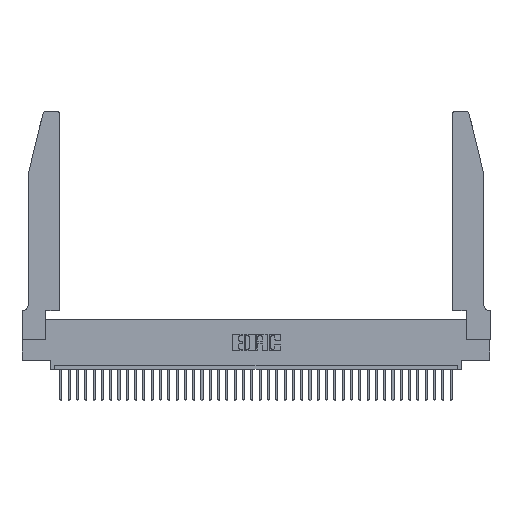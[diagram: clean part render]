
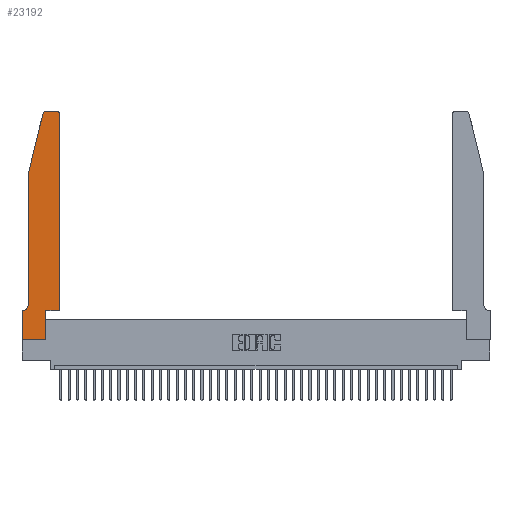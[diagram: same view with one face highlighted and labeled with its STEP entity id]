
A CAD part, top view. The second image highlights one B-rep face of the part: STEP entity #23192.
In plain terms, the highlighted planar face has unit normal (0, 0, 1).
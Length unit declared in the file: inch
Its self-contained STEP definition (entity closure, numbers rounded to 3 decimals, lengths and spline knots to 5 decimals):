
#135 = EDGE_CURVE ( 'NONE', #16836, #17390, #16397, .T. ) ;
#610 = DIRECTION ( 'NONE',  ( 1., 0., 0. ) ) ;
#1029 = DIRECTION ( 'NONE',  ( 0., -1., 0. ) ) ;
#2072 = ORIENTED_EDGE ( 'NONE', *, *, #16453, .T. ) ;
#3809 = EDGE_CURVE ( 'NONE', #31305, #38324, #21868, .T. ) ;
#4408 = AXIS2_PLACEMENT_3D ( 'NONE', #30358, #13214, #38181 ) ;
#4433 = ORIENTED_EDGE ( 'NONE', *, *, #30087, .T. ) ;
#4490 = EDGE_CURVE ( 'NONE', #38324, #21336, #21433, .T. ) ;
#5749 = ORIENTED_EDGE ( 'NONE', *, *, #23610, .T. ) ;
#5936 = LINE ( 'NONE', #21423, #18522 ) ;
#6411 = VECTOR ( 'NONE', #39731, 39.37008 ) ;
#6903 = VERTEX_POINT ( 'NONE', #28206 ) ;
#7872 = CARTESIAN_POINT ( 'NONE',  ( 0.25487, 2.72718, 0.37 ) ) ;
#8053 = CARTESIAN_POINT ( 'NONE',  ( 0., 0., 0.37 ) ) ;
#8839 = LINE ( 'NONE', #24676, #6411 ) ;
#9004 = VECTOR ( 'NONE', #610, 39.37008 ) ;
#9751 = CARTESIAN_POINT ( 'NONE',  ( 0.2605, 2.75, 0.37 ) ) ;
#9951 = AXIS2_PLACEMENT_3D ( 'NONE', #19405, #22533, #25153 ) ;
#10279 = VECTOR ( 'NONE', #39631, 39.37008 ) ;
#10837 = LINE ( 'NONE', #33483, #38509 ) ;
#10920 = FACE_OUTER_BOUND ( 'NONE', #16718, .T. ) ;
#11828 = EDGE_CURVE ( 'NONE', #39934, #39198, #5936, .T. ) ;
#13186 = VERTEX_POINT ( 'NONE', #14223 ) ;
#13214 = DIRECTION ( 'NONE',  ( 0., 0., -1. ) ) ;
#13774 = ORIENTED_EDGE ( 'NONE', *, *, #4490, .T. ) ;
#14223 = CARTESIAN_POINT ( 'NONE',  ( 0., 0.35, 0.37 ) ) ;
#15357 = CARTESIAN_POINT ( 'NONE',  ( 0.0755, 0.42, 0.37 ) ) ;
#16397 = CIRCLE ( 'NONE', #4408, 0.07 ) ;
#16434 = AXIS2_PLACEMENT_3D ( 'NONE', #36152, #20536, #32937 ) ;
#16453 = EDGE_CURVE ( 'NONE', #6903, #18025, #40066, .T. ) ;
#16718 = EDGE_LOOP ( 'NONE', ( #21951, #13774, #36897, #24852, #38712, #35125, #4433, #31146, #17960, #5749, #2072, #26581 ) ) ;
#16836 = VERTEX_POINT ( 'NONE', #15357 ) ;
#16858 = DIRECTION ( 'NONE',  ( 1., 0., 0. ) ) ;
#17140 = DIRECTION ( 'NONE',  ( 0., 0., 1. ) ) ;
#17390 = VERTEX_POINT ( 'NONE', #38244 ) ;
#17960 = ORIENTED_EDGE ( 'NONE', *, *, #11828, .T. ) ;
#18025 = VERTEX_POINT ( 'NONE', #33419 ) ;
#18165 = DIRECTION ( 'NONE',  ( 1., 0., 0. ) ) ;
#18201 = LINE ( 'NONE', #31940, #9004 ) ;
#18522 = VECTOR ( 'NONE', #24600, 39.37008 ) ;
#19405 = CARTESIAN_POINT ( 'NONE',  ( 0., 0.35, 0.37 ) ) ;
#19458 = VECTOR ( 'NONE', #34037, 39.37008 ) ;
#20536 = DIRECTION ( 'NONE',  ( 0., 0., 1. ) ) ;
#20901 = LINE ( 'NONE', #21155, #10279 ) ;
#21155 = CARTESIAN_POINT ( 'NONE',  ( 0.0755, 2., 0.37 ) ) ;
#21336 = VERTEX_POINT ( 'NONE', #7872 ) ;
#21423 = CARTESIAN_POINT ( 'NONE',  ( 0.2865, 0.35, 0.37 ) ) ;
#21433 = CIRCLE ( 'NONE', #16434, 0.03 ) ;
#21868 = LINE ( 'NONE', #9751, #19458 ) ;
#21951 = ORIENTED_EDGE ( 'NONE', *, *, #3809, .T. ) ;
#22125 = PLANE ( 'NONE',  #9951 ) ;
#22296 = CARTESIAN_POINT ( 'NONE',  ( 0., 0., 0.37 ) ) ;
#22533 = DIRECTION ( 'NONE',  ( 0., 0., 1. ) ) ;
#22954 = EDGE_CURVE ( 'NONE', #25829, #39934, #18201, .T. ) ;
#23192 = ADVANCED_FACE ( 'NONE', ( #10920 ), #22125, .T. ) ;
#23610 = EDGE_CURVE ( 'NONE', #39198, #6903, #10837, .T. ) ;
#23915 = DIRECTION ( 'NONE',  ( 0., 1., 0. ) ) ;
#24600 = DIRECTION ( 'NONE',  ( 0., 1., 0. ) ) ;
#24676 = CARTESIAN_POINT ( 'NONE',  ( 0.0755, 0.35, 0.37 ) ) ;
#24852 = ORIENTED_EDGE ( 'NONE', *, *, #33521, .T. ) ;
#25153 = DIRECTION ( 'NONE',  ( 1., 0., 0. ) ) ;
#25257 = EDGE_CURVE ( 'NONE', #21336, #33559, #32673, .T. ) ;
#25829 = VERTEX_POINT ( 'NONE', #8053 ) ;
#26127 = CARTESIAN_POINT ( 'NONE',  ( 0.284, 2.75, 0.37 ) ) ;
#26581 = ORIENTED_EDGE ( 'NONE', *, *, #28213, .T. ) ;
#27430 = VECTOR ( 'NONE', #23915, 39.37008 ) ;
#28206 = CARTESIAN_POINT ( 'NONE',  ( 0.4505, 0.35, 0.37 ) ) ;
#28213 = EDGE_CURVE ( 'NONE', #18025, #31305, #38814, .T. ) ;
#28311 = VECTOR ( 'NONE', #39854, 39.37008 ) ;
#30087 = EDGE_CURVE ( 'NONE', #13186, #25829, #34750, .T. ) ;
#30358 = CARTESIAN_POINT ( 'NONE',  ( 0.0055, 0.42, 0.37 ) ) ;
#30397 = CARTESIAN_POINT ( 'NONE',  ( 0.2865, 0.35, 0.37 ) ) ;
#31146 = ORIENTED_EDGE ( 'NONE', *, *, #22954, .T. ) ;
#31305 = VERTEX_POINT ( 'NONE', #38237 ) ;
#31940 = CARTESIAN_POINT ( 'NONE',  ( 0., 0., 0.37 ) ) ;
#32021 = CARTESIAN_POINT ( 'NONE',  ( 0.4205, 2.72, 0.37 ) ) ;
#32536 = CARTESIAN_POINT ( 'NONE',  ( 0.4505, 0.35, 0.37 ) ) ;
#32673 = LINE ( 'NONE', #39723, #28311 ) ;
#32674 = CARTESIAN_POINT ( 'NONE',  ( 0.0755, 2., 0.37 ) ) ;
#32719 = EDGE_CURVE ( 'NONE', #17390, #13186, #8839, .T. ) ;
#32937 = DIRECTION ( 'NONE',  ( 1., 0., 0. ) ) ;
#33419 = CARTESIAN_POINT ( 'NONE',  ( 0.4505, 2.72, 0.37 ) ) ;
#33483 = CARTESIAN_POINT ( 'NONE',  ( 0.4505, 0.35, 0.37 ) ) ;
#33521 = EDGE_CURVE ( 'NONE', #33559, #16836, #20901, .T. ) ;
#33559 = VERTEX_POINT ( 'NONE', #32674 ) ;
#33887 = CARTESIAN_POINT ( 'NONE',  ( 0.2865, 0., 0.37 ) ) ;
#34037 = DIRECTION ( 'NONE',  ( -1., 0., 0. ) ) ;
#34750 = LINE ( 'NONE', #22296, #39146 ) ;
#35125 = ORIENTED_EDGE ( 'NONE', *, *, #32719, .T. ) ;
#36152 = CARTESIAN_POINT ( 'NONE',  ( 0.284, 2.72, 0.37 ) ) ;
#36798 = AXIS2_PLACEMENT_3D ( 'NONE', #32021, #17140, #16858 ) ;
#36897 = ORIENTED_EDGE ( 'NONE', *, *, #25257, .T. ) ;
#38181 = DIRECTION ( 'NONE',  ( -1., 0., 0. ) ) ;
#38237 = CARTESIAN_POINT ( 'NONE',  ( 0.4205, 2.75, 0.37 ) ) ;
#38244 = CARTESIAN_POINT ( 'NONE',  ( 0.0055, 0.35, 0.37 ) ) ;
#38324 = VERTEX_POINT ( 'NONE', #26127 ) ;
#38509 = VECTOR ( 'NONE', #18165, 39.37008 ) ;
#38712 = ORIENTED_EDGE ( 'NONE', *, *, #135, .T. ) ;
#38814 = CIRCLE ( 'NONE', #36798, 0.03 ) ;
#39146 = VECTOR ( 'NONE', #1029, 39.37008 ) ;
#39198 = VERTEX_POINT ( 'NONE', #30397 ) ;
#39631 = DIRECTION ( 'NONE',  ( 0., -1., 0. ) ) ;
#39723 = CARTESIAN_POINT ( 'NONE',  ( 0.0755, 2., 0.37 ) ) ;
#39731 = DIRECTION ( 'NONE',  ( -1., 0., 0. ) ) ;
#39854 = DIRECTION ( 'NONE',  ( -0.239, -0.971, 0. ) ) ;
#39934 = VERTEX_POINT ( 'NONE', #33887 ) ;
#40066 = LINE ( 'NONE', #32536, #27430 ) ;
